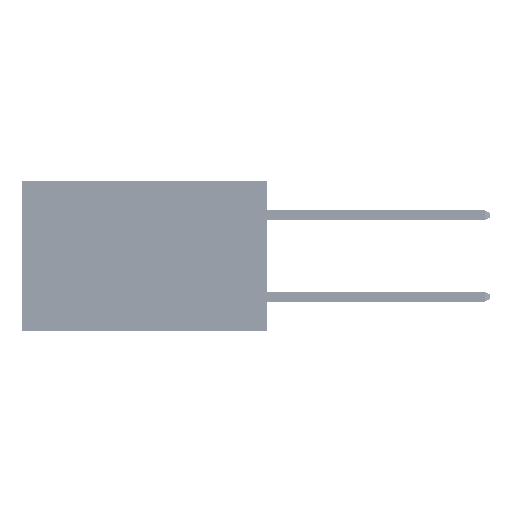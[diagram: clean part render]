
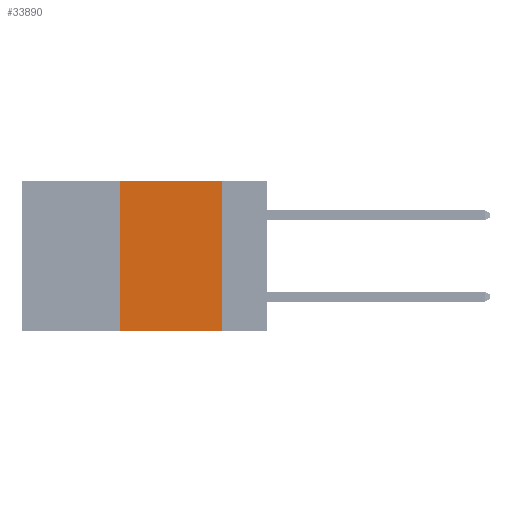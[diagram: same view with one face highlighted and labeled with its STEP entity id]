
A CAD part, left-side view. The second image highlights one B-rep face of the part: STEP entity #33890.
In plain terms, the highlighted planar face has unit normal (-1, 0, 0).
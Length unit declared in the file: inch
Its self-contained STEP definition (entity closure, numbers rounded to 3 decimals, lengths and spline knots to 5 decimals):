
#1402 = EDGE_CURVE ( 'NONE', #13715, #22377, #35598, .T. ) ;
#1443 = DIRECTION ( 'NONE',  ( 0., -1., 0. ) ) ;
#6329 = VERTEX_POINT ( 'NONE', #19322 ) ;
#6696 = CARTESIAN_POINT ( 'NONE',  ( 0., 0.36, -0.37 ) ) ;
#10965 = ORIENTED_EDGE ( 'NONE', *, *, #1402, .F. ) ;
#11337 = EDGE_CURVE ( 'NONE', #22377, #21464, #42044, .T. ) ;
#11650 = CARTESIAN_POINT ( 'NONE',  ( 0., 0.11, 0. ) ) ;
#11729 = FACE_OUTER_BOUND ( 'NONE', #32376, .T. ) ;
#13715 = VERTEX_POINT ( 'NONE', #6696 ) ;
#14894 = DIRECTION ( 'NONE',  ( 0., 0., -1. ) ) ;
#19226 = CARTESIAN_POINT ( 'NONE',  ( 0., 0.36, 0. ) ) ;
#19322 = CARTESIAN_POINT ( 'NONE',  ( 0., 0.11, -0.37 ) ) ;
#19483 = CARTESIAN_POINT ( 'NONE',  ( 0., 0.11, 0. ) ) ;
#20173 = LINE ( 'NONE', #23652, #38640 ) ;
#21464 = VERTEX_POINT ( 'NONE', #19483 ) ;
#22377 = VERTEX_POINT ( 'NONE', #39242 ) ;
#23652 = CARTESIAN_POINT ( 'NONE',  ( 0., 0.6, -0.37 ) ) ;
#23722 = VECTOR ( 'NONE', #1443, 39.37008 ) ;
#24513 = ORIENTED_EDGE ( 'NONE', *, *, #11337, .F. ) ;
#27022 = EDGE_CURVE ( 'NONE', #13715, #6329, #20173, .T. ) ;
#27341 = PLANE ( 'NONE',  #29590 ) ;
#28141 = DIRECTION ( 'NONE',  ( 1., 0., 0. ) ) ;
#29590 = AXIS2_PLACEMENT_3D ( 'NONE', #47999, #28141, #44518 ) ;
#30808 = DIRECTION ( 'NONE',  ( 0., 0., 1. ) ) ;
#32376 = EDGE_LOOP ( 'NONE', ( #37375, #24513, #10965, #36720 ) ) ;
#33890 = ADVANCED_FACE ( 'NONE', ( #11729 ), #27341, .F. ) ;
#35564 = LINE ( 'NONE', #11650, #37820 ) ;
#35598 = LINE ( 'NONE', #19226, #45239 ) ;
#36720 = ORIENTED_EDGE ( 'NONE', *, *, #27022, .T. ) ;
#37375 = ORIENTED_EDGE ( 'NONE', *, *, #44105, .F. ) ;
#37820 = VECTOR ( 'NONE', #14894, 39.37008 ) ;
#38640 = VECTOR ( 'NONE', #43801, 39.37008 ) ;
#39242 = CARTESIAN_POINT ( 'NONE',  ( 0., 0.36, 0. ) ) ;
#42044 = LINE ( 'NONE', #45806, #23722 ) ;
#43801 = DIRECTION ( 'NONE',  ( 0., -1., 0. ) ) ;
#44105 = EDGE_CURVE ( 'NONE', #21464, #6329, #35564, .T. ) ;
#44518 = DIRECTION ( 'NONE',  ( 0., 0., -1. ) ) ;
#45239 = VECTOR ( 'NONE', #30808, 39.37008 ) ;
#45806 = CARTESIAN_POINT ( 'NONE',  ( 0., 0.6, 0. ) ) ;
#47999 = CARTESIAN_POINT ( 'NONE',  ( 0., 0.6, 0. ) ) ;
